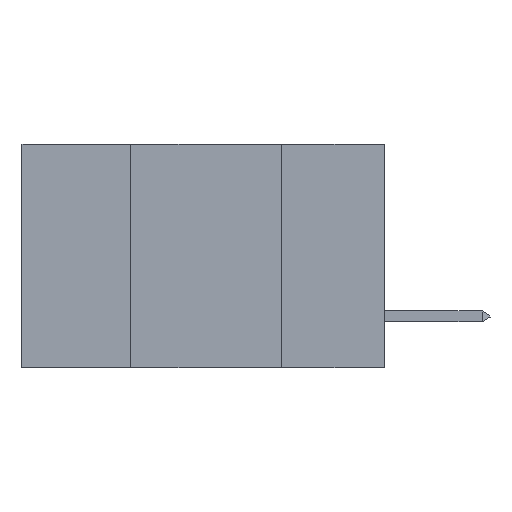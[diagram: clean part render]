
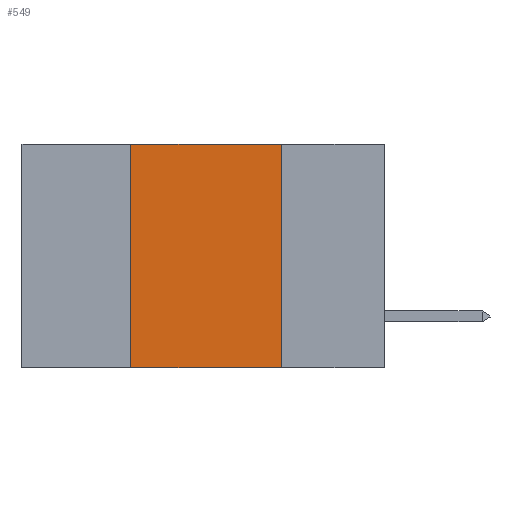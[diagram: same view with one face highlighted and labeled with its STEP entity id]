
A CAD part, left-side view. The second image highlights one B-rep face of the part: STEP entity #549.
In plain terms, the highlighted planar face has unit normal (-1, 0, 0).
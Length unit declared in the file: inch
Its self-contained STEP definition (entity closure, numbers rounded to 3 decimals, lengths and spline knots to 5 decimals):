
#236 = VERTEX_POINT ( 'NONE', #1910 ) ;
#549 = ADVANCED_FACE ( 'NONE', ( #8009 ), #17248, .F. ) ;
#1033 = CARTESIAN_POINT ( 'NONE',  ( 0., 0.6, -0.37 ) ) ;
#1332 = CARTESIAN_POINT ( 'NONE',  ( 0., 0.17, -0.37 ) ) ;
#1910 = CARTESIAN_POINT ( 'NONE',  ( 0., 0.42, 0. ) ) ;
#3644 = VERTEX_POINT ( 'NONE', #1332 ) ;
#3683 = DIRECTION ( 'NONE',  ( 0., 0., -1. ) ) ;
#6740 = AXIS2_PLACEMENT_3D ( 'NONE', #16589, #15563, #3683 ) ;
#7180 = CARTESIAN_POINT ( 'NONE',  ( 0., 0.17, 0. ) ) ;
#7924 = EDGE_CURVE ( 'NONE', #12408, #3644, #18360, .T. ) ;
#8009 = FACE_OUTER_BOUND ( 'NONE', #13108, .T. ) ;
#9228 = CARTESIAN_POINT ( 'NONE',  ( 0., 0.42, 0. ) ) ;
#9364 = VECTOR ( 'NONE', #12556, 39.37008 ) ;
#11473 = DIRECTION ( 'NONE',  ( 0., -1., 0. ) ) ;
#12286 = VERTEX_POINT ( 'NONE', #7180 ) ;
#12408 = VERTEX_POINT ( 'NONE', #19277 ) ;
#12556 = DIRECTION ( 'NONE',  ( 0., 0., 1. ) ) ;
#12978 = ORIENTED_EDGE ( 'NONE', *, *, #18939, .F. ) ;
#13108 = EDGE_LOOP ( 'NONE', ( #13423, #12978, #13802, #13525 ) ) ;
#13423 = ORIENTED_EDGE ( 'NONE', *, *, #13551, .F. ) ;
#13525 = ORIENTED_EDGE ( 'NONE', *, *, #7924, .T. ) ;
#13551 = EDGE_CURVE ( 'NONE', #12286, #3644, #18477, .T. ) ;
#13802 = ORIENTED_EDGE ( 'NONE', *, *, #21357, .F. ) ;
#13959 = DIRECTION ( 'NONE',  ( 0., 0., -1. ) ) ;
#14239 = VECTOR ( 'NONE', #11473, 39.37008 ) ;
#15563 = DIRECTION ( 'NONE',  ( 1., 0., 0. ) ) ;
#15692 = CARTESIAN_POINT ( 'NONE',  ( 0., 0.17, 0. ) ) ;
#16589 = CARTESIAN_POINT ( 'NONE',  ( 0., 0.6, 0. ) ) ;
#17248 = PLANE ( 'NONE',  #6740 ) ;
#17818 = LINE ( 'NONE', #9228, #9364 ) ;
#17956 = VECTOR ( 'NONE', #13959, 39.37008 ) ;
#18360 = LINE ( 'NONE', #1033, #21288 ) ;
#18477 = LINE ( 'NONE', #15692, #17956 ) ;
#18939 = EDGE_CURVE ( 'NONE', #236, #12286, #19224, .T. ) ;
#19224 = LINE ( 'NONE', #19849, #14239 ) ;
#19277 = CARTESIAN_POINT ( 'NONE',  ( 0., 0.42, -0.37 ) ) ;
#19568 = DIRECTION ( 'NONE',  ( 0., -1., 0. ) ) ;
#19849 = CARTESIAN_POINT ( 'NONE',  ( 0., 0.6, 0. ) ) ;
#21288 = VECTOR ( 'NONE', #19568, 39.37008 ) ;
#21357 = EDGE_CURVE ( 'NONE', #12408, #236, #17818, .T. ) ;
